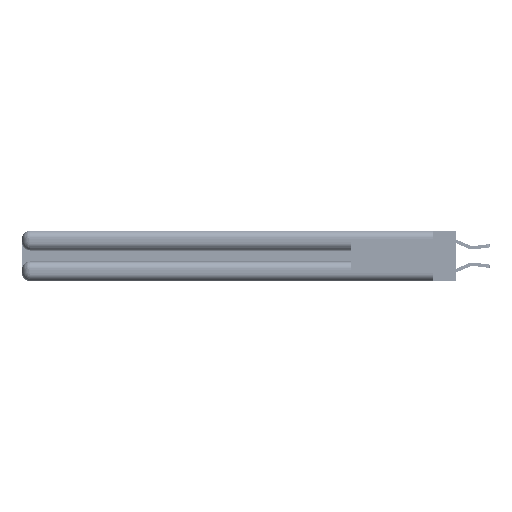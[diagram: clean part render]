
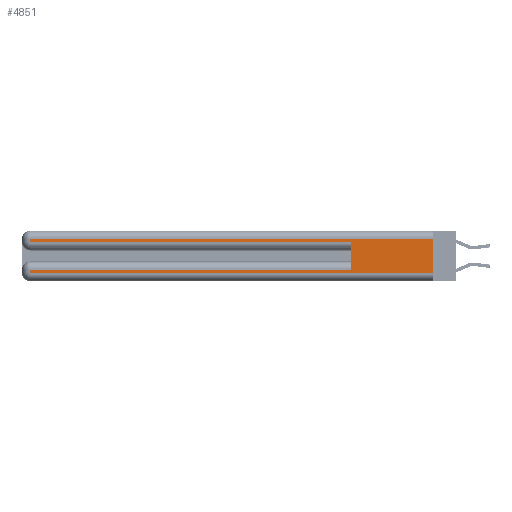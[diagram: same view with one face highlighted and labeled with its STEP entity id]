
A CAD part, left-side view. The second image highlights one B-rep face of the part: STEP entity #4851.
In plain terms, the highlighted planar face has unit normal (-1, 0, 0).
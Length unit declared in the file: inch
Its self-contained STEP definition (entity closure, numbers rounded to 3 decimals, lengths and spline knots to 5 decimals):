
#375 = LINE ( 'NONE', #4227, #30150 ) ;
#547 = CARTESIAN_POINT ( 'NONE',  ( 0., 2.94, 0.06 ) ) ;
#602 = VERTEX_POINT ( 'NONE', #21299 ) ;
#1600 = VECTOR ( 'NONE', #13169, 39.37008 ) ;
#1703 = DIRECTION ( 'NONE',  ( 0., -1., 0. ) ) ;
#1948 = CARTESIAN_POINT ( 'NONE',  ( 0., 0.6, 0.085 ) ) ;
#1969 = ORIENTED_EDGE ( 'NONE', *, *, #23978, .T. ) ;
#2014 = LINE ( 'NONE', #30230, #24119 ) ;
#2211 = VERTEX_POINT ( 'NONE', #25201 ) ;
#2784 = EDGE_LOOP ( 'NONE', ( #12925, #30667, #34876, #7364, #5141, #1969, #7973, #19123 ) ) ;
#4227 = CARTESIAN_POINT ( 'NONE',  ( 0., 0., 0.37 ) ) ;
#4648 = CARTESIAN_POINT ( 'NONE',  ( 0., 0., 0.06 ) ) ;
#4851 = ADVANCED_FACE ( 'NONE', ( #35389 ), #20711, .F. ) ;
#5141 = ORIENTED_EDGE ( 'NONE', *, *, #33539, .F. ) ;
#7150 = DIRECTION ( 'NONE',  ( 0., 0., -1. ) ) ;
#7307 = VERTEX_POINT ( 'NONE', #547 ) ;
#7364 = ORIENTED_EDGE ( 'NONE', *, *, #19418, .T. ) ;
#7973 = ORIENTED_EDGE ( 'NONE', *, *, #22059, .T. ) ;
#9347 = VECTOR ( 'NONE', #1703, 39.37008 ) ;
#10468 = CARTESIAN_POINT ( 'NONE',  ( 0., 0.6, 0.145 ) ) ;
#10495 = DIRECTION ( 'NONE',  ( 0., 0., -1. ) ) ;
#11093 = VERTEX_POINT ( 'NONE', #1948 ) ;
#11182 = DIRECTION ( 'NONE',  ( 0., 1., 0. ) ) ;
#12505 = CARTESIAN_POINT ( 'NONE',  ( 0., 2.94, 0.085 ) ) ;
#12925 = ORIENTED_EDGE ( 'NONE', *, *, #27573, .F. ) ;
#13169 = DIRECTION ( 'NONE',  ( 0., 0., -1. ) ) ;
#15092 = VERTEX_POINT ( 'NONE', #17962 ) ;
#16284 = DIRECTION ( 'NONE',  ( 0., 0., 1. ) ) ;
#16477 = VECTOR ( 'NONE', #36986, 39.37008 ) ;
#16483 = CARTESIAN_POINT ( 'NONE',  ( 0., 0.6, 0.285 ) ) ;
#17891 = LINE ( 'NONE', #30400, #1600 ) ;
#17955 = DIRECTION ( 'NONE',  ( 0., 0., -1. ) ) ;
#17962 = CARTESIAN_POINT ( 'NONE',  ( 0., 0., 0.06 ) ) ;
#18025 = CARTESIAN_POINT ( 'NONE',  ( 0., 2.94, 0.285 ) ) ;
#18832 = LINE ( 'NONE', #30595, #27340 ) ;
#18994 = VERTEX_POINT ( 'NONE', #18025 ) ;
#19123 = ORIENTED_EDGE ( 'NONE', *, *, #22781, .T. ) ;
#19418 = EDGE_CURVE ( 'NONE', #18994, #29570, #31699, .T. ) ;
#19874 = CARTESIAN_POINT ( 'NONE',  ( 0., 0., 0.285 ) ) ;
#20711 = PLANE ( 'NONE',  #21967 ) ;
#21299 = CARTESIAN_POINT ( 'NONE',  ( 0., 2.94, 0.31 ) ) ;
#21908 = VECTOR ( 'NONE', #16284, 39.37008 ) ;
#21934 = VERTEX_POINT ( 'NONE', #12505 ) ;
#21967 = AXIS2_PLACEMENT_3D ( 'NONE', #29342, #35078, #17955 ) ;
#22059 = EDGE_CURVE ( 'NONE', #21934, #7307, #18832, .T. ) ;
#22438 = LINE ( 'NONE', #36879, #29124 ) ;
#22781 = EDGE_CURVE ( 'NONE', #7307, #15092, #32259, .T. ) ;
#23267 = EDGE_CURVE ( 'NONE', #602, #18994, #17891, .T. ) ;
#23978 = EDGE_CURVE ( 'NONE', #11093, #21934, #2014, .T. ) ;
#24119 = VECTOR ( 'NONE', #35951, 39.37008 ) ;
#25201 = CARTESIAN_POINT ( 'NONE',  ( 0., 0., 0.31 ) ) ;
#27340 = VECTOR ( 'NONE', #10495, 39.37008 ) ;
#27573 = EDGE_CURVE ( 'NONE', #2211, #15092, #375, .T. ) ;
#28995 = EDGE_CURVE ( 'NONE', #2211, #602, #22438, .T. ) ;
#29124 = VECTOR ( 'NONE', #11182, 39.37008 ) ;
#29342 = CARTESIAN_POINT ( 'NONE',  ( 0., 0., 0.37 ) ) ;
#29570 = VERTEX_POINT ( 'NONE', #16483 ) ;
#30150 = VECTOR ( 'NONE', #7150, 39.37008 ) ;
#30230 = CARTESIAN_POINT ( 'NONE',  ( 0., 0., 0.085 ) ) ;
#30400 = CARTESIAN_POINT ( 'NONE',  ( 0., 2.94, 0.37 ) ) ;
#30422 = LINE ( 'NONE', #10468, #21908 ) ;
#30595 = CARTESIAN_POINT ( 'NONE',  ( 0., 2.94, 0.37 ) ) ;
#30667 = ORIENTED_EDGE ( 'NONE', *, *, #28995, .T. ) ;
#31699 = LINE ( 'NONE', #19874, #16477 ) ;
#32259 = LINE ( 'NONE', #4648, #9347 ) ;
#33539 = EDGE_CURVE ( 'NONE', #11093, #29570, #30422, .T. ) ;
#34876 = ORIENTED_EDGE ( 'NONE', *, *, #23267, .T. ) ;
#35078 = DIRECTION ( 'NONE',  ( 1., 0., 0. ) ) ;
#35389 = FACE_OUTER_BOUND ( 'NONE', #2784, .T. ) ;
#35951 = DIRECTION ( 'NONE',  ( 0., 1., 0. ) ) ;
#36879 = CARTESIAN_POINT ( 'NONE',  ( 0., 0., 0.31 ) ) ;
#36986 = DIRECTION ( 'NONE',  ( 0., -1., 0. ) ) ;
